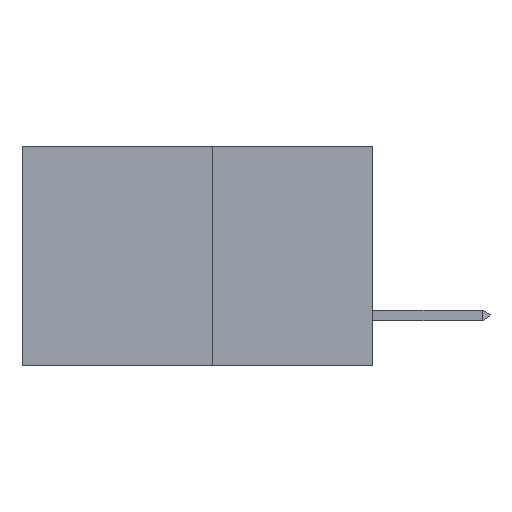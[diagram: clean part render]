
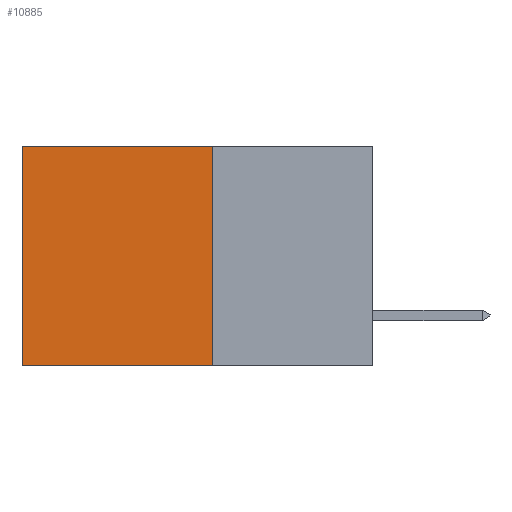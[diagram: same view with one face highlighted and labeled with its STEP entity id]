
A CAD part, left-side view. The second image highlights one B-rep face of the part: STEP entity #10885.
In plain terms, the highlighted planar face has unit normal (-1, 0, 0).
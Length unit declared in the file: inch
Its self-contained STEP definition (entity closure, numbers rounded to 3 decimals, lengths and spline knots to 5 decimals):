
#51 = ORIENTED_EDGE ( 'NONE', *, *, #9611, .F. ) ;
#1146 = VERTEX_POINT ( 'NONE', #11717 ) ;
#1334 = EDGE_LOOP ( 'NONE', ( #2557, #51, #1598, #4867 ) ) ;
#1374 = DIRECTION ( 'NONE',  ( 0., 0., -1. ) ) ;
#1492 = CARTESIAN_POINT ( 'NONE',  ( 0.277, 0.59, 0. ) ) ;
#1598 = ORIENTED_EDGE ( 'NONE', *, *, #10867, .F. ) ;
#2197 = CARTESIAN_POINT ( 'NONE',  ( 0.277, 0.27, -0.37 ) ) ;
#2508 = CARTESIAN_POINT ( 'NONE',  ( 0.277, 0.59, -0.37 ) ) ;
#2557 = ORIENTED_EDGE ( 'NONE', *, *, #8002, .T. ) ;
#3342 = CARTESIAN_POINT ( 'NONE',  ( 0.277, 0.27, -0.37 ) ) ;
#4240 = DIRECTION ( 'NONE',  ( 0., 1., 0. ) ) ;
#4759 = LINE ( 'NONE', #11570, #14469 ) ;
#4764 = AXIS2_PLACEMENT_3D ( 'NONE', #3342, #7036, #15499 ) ;
#4867 = ORIENTED_EDGE ( 'NONE', *, *, #6012, .T. ) ;
#5835 = VECTOR ( 'NONE', #11935, 39.37008 ) ;
#6012 = EDGE_CURVE ( 'NONE', #14474, #9433, #4759, .T. ) ;
#6991 = LINE ( 'NONE', #2508, #13461 ) ;
#7036 = DIRECTION ( 'NONE',  ( 1., 0., 0. ) ) ;
#7868 = VECTOR ( 'NONE', #8189, 39.37008 ) ;
#8002 = EDGE_CURVE ( 'NONE', #9433, #1146, #6991, .T. ) ;
#8189 = DIRECTION ( 'NONE',  ( 0., 0., -1. ) ) ;
#8246 = FACE_OUTER_BOUND ( 'NONE', #1334, .T. ) ;
#9433 = VERTEX_POINT ( 'NONE', #1492 ) ;
#9611 = EDGE_CURVE ( 'NONE', #9641, #1146, #12314, .T. ) ;
#9641 = VERTEX_POINT ( 'NONE', #2197 ) ;
#10867 = EDGE_CURVE ( 'NONE', #14474, #9641, #11133, .T. ) ;
#10885 = ADVANCED_FACE ( 'NONE', ( #8246 ), #14309, .F. ) ;
#10987 = CARTESIAN_POINT ( 'NONE',  ( 0.277, 0.27, 0. ) ) ;
#11133 = LINE ( 'NONE', #14255, #7868 ) ;
#11570 = CARTESIAN_POINT ( 'NONE',  ( 0.277, 0.27, 0. ) ) ;
#11717 = CARTESIAN_POINT ( 'NONE',  ( 0.277, 0.59, -0.37 ) ) ;
#11935 = DIRECTION ( 'NONE',  ( 0., 1., 0. ) ) ;
#12314 = LINE ( 'NONE', #15432, #5835 ) ;
#13461 = VECTOR ( 'NONE', #1374, 39.37008 ) ;
#14255 = CARTESIAN_POINT ( 'NONE',  ( 0.277, 0.27, -0.37 ) ) ;
#14309 = PLANE ( 'NONE',  #4764 ) ;
#14469 = VECTOR ( 'NONE', #4240, 39.37008 ) ;
#14474 = VERTEX_POINT ( 'NONE', #10987 ) ;
#15432 = CARTESIAN_POINT ( 'NONE',  ( 0.277, 0.27, -0.37 ) ) ;
#15499 = DIRECTION ( 'NONE',  ( 0., 0., -1. ) ) ;
